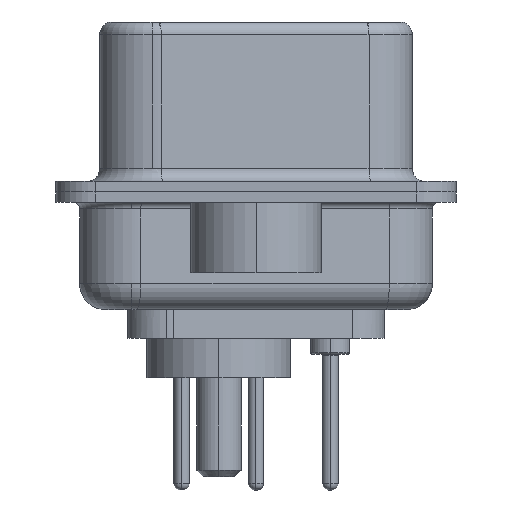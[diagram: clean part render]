
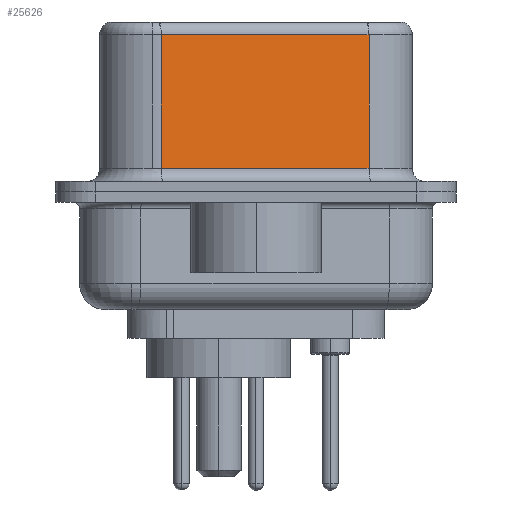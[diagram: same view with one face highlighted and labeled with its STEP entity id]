
A CAD part, left-side view. The second image highlights one B-rep face of the part: STEP entity #25626.
In plain terms, the highlighted planar face has unit normal (-0.985, -0.174, 0).
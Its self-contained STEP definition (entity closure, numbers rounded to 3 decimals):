
#338 = ORIENTED_EDGE ( 'NONE', *, *, #21291, .T. ) ;
#374 = DIRECTION ( 'NONE',  ( 0., 0., -1. ) ) ;
#3587 = DIRECTION ( 'NONE',  ( -0.174, 0.985, 0. ) ) ;
#4013 = LINE ( 'NONE', #20932, #15437 ) ;
#4493 = VERTEX_POINT ( 'NONE', #14400 ) ;
#4992 = VECTOR ( 'NONE', #7627, 1000. ) ;
#5126 = VERTEX_POINT ( 'NONE', #11474 ) ;
#7627 = DIRECTION ( 'NONE',  ( 0., 0., -1. ) ) ;
#7880 = CARTESIAN_POINT ( 'NONE',  ( 5.132, -4.322, 0.9 ) ) ;
#8184 = EDGE_LOOP ( 'NONE', ( #14244, #20007, #24298, #338 ) ) ;
#8606 = CARTESIAN_POINT ( 'NONE',  ( 5.132, -4.322, 6.52 ) ) ;
#8790 = VECTOR ( 'NONE', #9952, 1000. ) ;
#9277 = VECTOR ( 'NONE', #3587, 1000. ) ;
#9952 = DIRECTION ( 'NONE',  ( 0.174, -0.985, 0. ) ) ;
#10083 = AXIS2_PLACEMENT_3D ( 'NONE', #8606, #23390, #11091 ) ;
#11091 = DIRECTION ( 'NONE',  ( -0.174, 0.985, 0. ) ) ;
#11474 = CARTESIAN_POINT ( 'NONE',  ( 3.73, 3.628, 6.02 ) ) ;
#11833 = CARTESIAN_POINT ( 'NONE',  ( 5.132, -4.322, 6.02 ) ) ;
#14206 = CARTESIAN_POINT ( 'NONE',  ( 5.132, -4.322, 0.9 ) ) ;
#14244 = ORIENTED_EDGE ( 'NONE', *, *, #24205, .F. ) ;
#14400 = CARTESIAN_POINT ( 'NONE',  ( 3.73, 3.628, 0.9 ) ) ;
#15135 = LINE ( 'NONE', #19959, #4992 ) ;
#15437 = VECTOR ( 'NONE', #374, 1000. ) ;
#15677 = FACE_OUTER_BOUND ( 'NONE', #8184, .T. ) ;
#15754 = CARTESIAN_POINT ( 'NONE',  ( 5.132, -4.322, 6.02 ) ) ;
#17061 = VERTEX_POINT ( 'NONE', #11833 ) ;
#17687 = EDGE_CURVE ( 'NONE', #17061, #5126, #25720, .T. ) ;
#19959 = CARTESIAN_POINT ( 'NONE',  ( 3.73, 3.628, 6.52 ) ) ;
#20007 = ORIENTED_EDGE ( 'NONE', *, *, #17687, .T. ) ;
#20932 = CARTESIAN_POINT ( 'NONE',  ( 5.132, -4.322, 6.52 ) ) ;
#20958 = PLANE ( 'NONE',  #10083 ) ;
#21291 = EDGE_CURVE ( 'NONE', #4493, #24056, #25231, .T. ) ;
#23390 = DIRECTION ( 'NONE',  ( 0.985, 0.174, 0. ) ) ;
#23905 = EDGE_CURVE ( 'NONE', #5126, #4493, #15135, .T. ) ;
#24056 = VERTEX_POINT ( 'NONE', #14206 ) ;
#24205 = EDGE_CURVE ( 'NONE', #17061, #24056, #4013, .T. ) ;
#24298 = ORIENTED_EDGE ( 'NONE', *, *, #23905, .T. ) ;
#25231 = LINE ( 'NONE', #7880, #8790 ) ;
#25626 = ADVANCED_FACE ( 'NONE', ( #15677 ), #20958, .F. ) ;
#25720 = LINE ( 'NONE', #15754, #9277 ) ;
